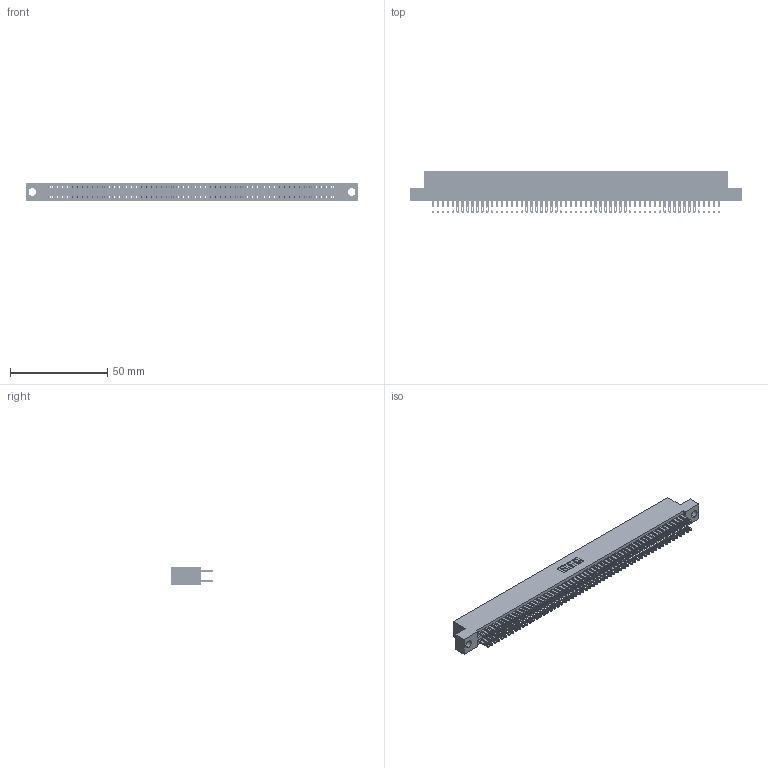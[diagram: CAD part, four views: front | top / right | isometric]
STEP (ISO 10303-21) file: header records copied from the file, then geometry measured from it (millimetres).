
FILE_DESCRIPTION (( 'STEP AP203' ), '1' );
FILE_NAME ('345-118-500-204.STEP', '2021-05-25T16:01:09', ( '' ), ( '' ), 'SwSTEP 2.0', 'SolidWorks 2020', '' );
FILE_SCHEMA (( 'CONFIG_CONTROL_DESIGN' ));
Length unit declared in the file: inch
Products named in the file (3): 345-118-500-204; 345 Part_Flush Mounting Lugs - 0.156 Dia-TI; 345-292-001_345-293-100
Assembly tree (119 placements, depth 2):
  345-118-500-204
    345 Part_Flush Mounting Lugs - 0.156 Dia-TI
    345-292-001_345-293-100  x118
Bounding box: 171.07 x 21.51 x 9.4 mm (x, y, z)
Volume: 17030.3 mm3; surface area: 26558 mm2
Topology: 119 solids, 119 shells, 5568 faces, 17015 edges, 11342 vertices
Faces by surface type: plane 3280, cylinder 2288
Entity records: 44353 total; most frequent: CARTESIAN_POINT 7422, ORIENTED_EDGE 7354, DIRECTION 6525, EDGE_CURVE 3677, VECTOR 3305, LINE 3305, VERTEX_POINT 2450, AXIS2_PLACEMENT_3D 1610
